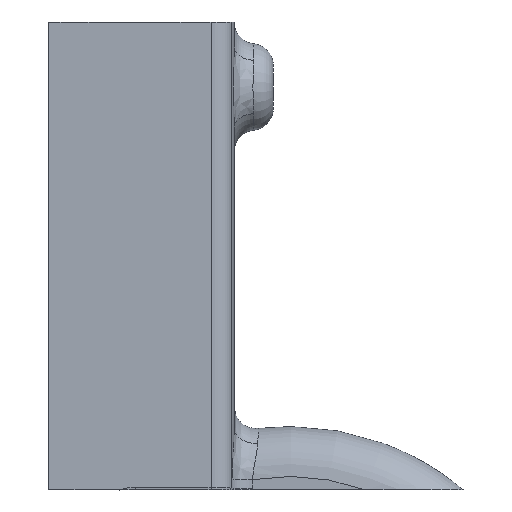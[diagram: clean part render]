
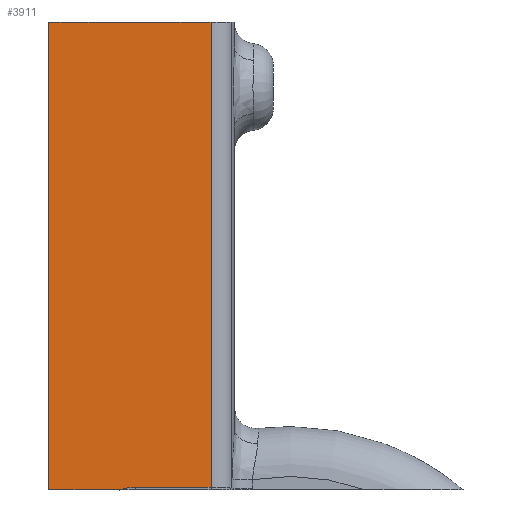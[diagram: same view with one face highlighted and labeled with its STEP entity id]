
A CAD part, left-side view. The second image highlights one B-rep face of the part: STEP entity #3911.
In plain terms, the highlighted planar face has unit normal (-1, 0, 0).
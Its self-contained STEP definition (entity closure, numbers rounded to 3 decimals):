
#121 = CARTESIAN_POINT ( 'NONE',  ( -66.655, 14.938, 31.739 ) ) ;
#130 = AXIS2_PLACEMENT_3D ( 'NONE', #4001, #3564, #3543 ) ;
#161 = EDGE_CURVE ( 'NONE', #691, #4727, #4114, .T. ) ;
#308 = ORIENTED_EDGE ( 'NONE', *, *, #3215, .T. ) ;
#359 = CARTESIAN_POINT ( 'NONE',  ( -66.655, -8.53, 31.739 ) ) ;
#550 = CARTESIAN_POINT ( 'NONE',  ( -66.655, -13.175, 31.739 ) ) ;
#564 = EDGE_CURVE ( 'NONE', #691, #5321, #4891, .T. ) ;
#586 = EDGE_CURVE ( 'NONE', #4818, #4833, #4742, .T. ) ;
#639 = CARTESIAN_POINT ( 'NONE',  ( -66.655, 12.158, -76.26 ) ) ;
#691 = VERTEX_POINT ( 'NONE', #5725 ) ;
#814 = DIRECTION ( 'NONE',  ( 0., 1., 0. ) ) ;
#878 = DIRECTION ( 'NONE',  ( 0., 1., 0. ) ) ;
#1080 = VECTOR ( 'NONE', #4116, 1000. ) ;
#1129 = CARTESIAN_POINT ( 'NONE',  ( -66.655, 4.281, -75.639 ) ) ;
#1176 = CARTESIAN_POINT ( 'NONE',  ( -66.655, 24.278, 31.739 ) ) ;
#1396 = ORIENTED_EDGE ( 'NONE', *, *, #2938, .T. ) ;
#1749 = CARTESIAN_POINT ( 'NONE',  ( -66.655, 24.278, -76.26 ) ) ;
#1950 = CARTESIAN_POINT ( 'NONE',  ( -66.655, 15.287, 31.739 ) ) ;
#2176 = VECTOR ( 'NONE', #3723, 1000. ) ;
#2193 = VECTOR ( 'NONE', #4052, 1000. ) ;
#2329 = LINE ( 'NONE', #3741, #5655 ) ;
#2441 = ORIENTED_EDGE ( 'NONE', *, *, #2948, .T. ) ;
#2554 = VERTEX_POINT ( 'NONE', #550 ) ;
#2839 = ORIENTED_EDGE ( 'NONE', *, *, #161, .T. ) ;
#2938 = EDGE_CURVE ( 'NONE', #4727, #3335, #3788, .T. ) ;
#2948 = EDGE_CURVE ( 'NONE', #3335, #2554, #4890, .T. ) ;
#2959 = EDGE_CURVE ( 'NONE', #2554, #4818, #3640, .T. ) ;
#3068 = CARTESIAN_POINT ( 'NONE',  ( -66.655, -13.175, -75.639 ) ) ;
#3204 = EDGE_CURVE ( 'NONE', #4833, #4775, #2329, .T. ) ;
#3206 = EDGE_CURVE ( 'NONE', #4775, #3801, #4776, .T. ) ;
#3210 = CARTESIAN_POINT ( 'NONE',  ( -66.655, 4.281, -75.639 ) ) ;
#3215 = EDGE_CURVE ( 'NONE', #3801, #4969, #4678, .T. ) ;
#3223 = EDGE_CURVE ( 'NONE', #5321, #4969, #3482, .T. ) ;
#3335 = VERTEX_POINT ( 'NONE', #3068 ) ;
#3345 = CARTESIAN_POINT ( 'NONE',  ( -66.655, 7.344, -76.055 ) ) ;
#3377 = CARTESIAN_POINT ( 'NONE',  ( -66.655, 5.836, -75.716 ) ) ;
#3393 = CARTESIAN_POINT ( 'NONE',  ( -66.655, 6.97, -75.955 ) ) ;
#3396 = CARTESIAN_POINT ( 'NONE',  ( -66.655, 7.949, -76.26 ) ) ;
#3418 = CARTESIAN_POINT ( 'NONE',  ( -66.655, 5.066, -75.639 ) ) ;
#3482 = LINE ( 'NONE', #3704, #5463 ) ;
#3543 = DIRECTION ( 'NONE',  ( 0., 0., -1. ) ) ;
#3548 = CARTESIAN_POINT ( 'NONE',  ( -66.655, 7.792, -76.204 ) ) ;
#3564 = DIRECTION ( 'NONE',  ( 1., 0., 0. ) ) ;
#3591 = CARTESIAN_POINT ( 'NONE',  ( -66.655, 7.871, -76.232 ) ) ;
#3640 = LINE ( 'NONE', #4106, #2193 ) ;
#3671 = DIRECTION ( 'NONE',  ( 0., 0., 1. ) ) ;
#3689 = CARTESIAN_POINT ( 'NONE',  ( -66.655, -8.53, 31.739 ) ) ;
#3704 = CARTESIAN_POINT ( 'NONE',  ( -66.655, 24.278, -343.011 ) ) ;
#3723 = DIRECTION ( 'NONE',  ( 0., 1., 0. ) ) ;
#3740 = DIRECTION ( 'NONE',  ( 0., 1., 0. ) ) ;
#3741 = CARTESIAN_POINT ( 'NONE',  ( -66.655, -8.53, 31.739 ) ) ;
#3775 = CARTESIAN_POINT ( 'NONE',  ( -66.655, -8.53, 31.739 ) ) ;
#3788 = LINE ( 'NONE', #4192, #4785 ) ;
#3801 = VERTEX_POINT ( 'NONE', #1950 ) ;
#3827 = DIRECTION ( 'NONE',  ( 0., 1., 0. ) ) ;
#3911 = ADVANCED_FACE ( 'NONE', ( #4843 ), #4018, .F. ) ;
#4001 = CARTESIAN_POINT ( 'NONE',  ( -66.655, 12.158, -321.506 ) ) ;
#4018 = PLANE ( 'NONE',  #130 ) ;
#4052 = DIRECTION ( 'NONE',  ( 0., 1., 0. ) ) ;
#4106 = CARTESIAN_POINT ( 'NONE',  ( -66.655, -8.53, 31.739 ) ) ;
#4114 = B_SPLINE_CURVE_WITH_KNOTS ( 'NONE', 3,
 ( #3396, #3591, #3548, #3345, #3393, #3377, #3418, #3210 ),
 .UNSPECIFIED., .F., .F.,
 ( 4, 2, 2, 4 ),
 ( 0.006, 0.006, 0.007, 0.009 ),
 .UNSPECIFIED. ) ;
#4116 = DIRECTION ( 'NONE',  ( 0., 0., 1. ) ) ;
#4161 = CARTESIAN_POINT ( 'NONE',  ( -66.655, -13.175, 31.739 ) ) ;
#4174 = DIRECTION ( 'NONE',  ( 0., -1., 0. ) ) ;
#4192 = CARTESIAN_POINT ( 'NONE',  ( -66.655, 12.158, -75.639 ) ) ;
#4554 = ORIENTED_EDGE ( 'NONE', *, *, #586, .T. ) ;
#4591 = ORIENTED_EDGE ( 'NONE', *, *, #2959, .T. ) ;
#4637 = VECTOR ( 'NONE', #878, 1000. ) ;
#4652 = ORIENTED_EDGE ( 'NONE', *, *, #3223, .F. ) ;
#4678 = LINE ( 'NONE', #3689, #2176 ) ;
#4727 = VERTEX_POINT ( 'NONE', #1129 ) ;
#4742 = LINE ( 'NONE', #359, #4637 ) ;
#4758 = EDGE_LOOP ( 'NONE', ( #4915, #2839, #1396, #2441, #4591, #4554, #5443, #5200, #308, #4652 ) ) ;
#4775 = VERTEX_POINT ( 'NONE', #121 ) ;
#4776 = LINE ( 'NONE', #3775, #5562 ) ;
#4785 = VECTOR ( 'NONE', #4174, 1000. ) ;
#4818 = VERTEX_POINT ( 'NONE', #5507 ) ;
#4830 = CARTESIAN_POINT ( 'NONE',  ( -66.655, -5.927, 31.739 ) ) ;
#4833 = VERTEX_POINT ( 'NONE', #4830 ) ;
#4838 = VECTOR ( 'NONE', #814, 1000. ) ;
#4843 = FACE_OUTER_BOUND ( 'NONE', #4758, .T. ) ;
#4890 = LINE ( 'NONE', #4161, #1080 ) ;
#4891 = LINE ( 'NONE', #639, #4838 ) ;
#4915 = ORIENTED_EDGE ( 'NONE', *, *, #564, .F. ) ;
#4969 = VERTEX_POINT ( 'NONE', #1176 ) ;
#5200 = ORIENTED_EDGE ( 'NONE', *, *, #3206, .T. ) ;
#5321 = VERTEX_POINT ( 'NONE', #1749 ) ;
#5443 = ORIENTED_EDGE ( 'NONE', *, *, #3204, .T. ) ;
#5463 = VECTOR ( 'NONE', #3671, 1000. ) ;
#5507 = CARTESIAN_POINT ( 'NONE',  ( -66.655, -6.275, 31.739 ) ) ;
#5562 = VECTOR ( 'NONE', #3827, 1000. ) ;
#5655 = VECTOR ( 'NONE', #3740, 1000. ) ;
#5725 = CARTESIAN_POINT ( 'NONE',  ( -66.655, 7.949, -76.26 ) ) ;
